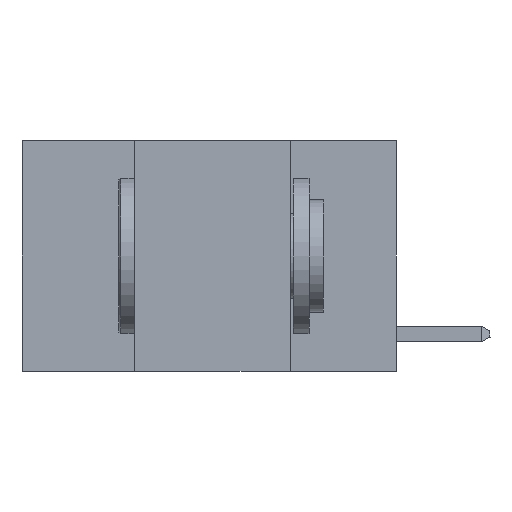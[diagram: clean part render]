
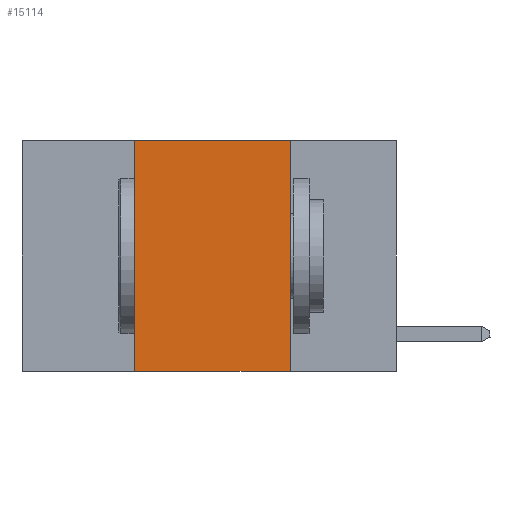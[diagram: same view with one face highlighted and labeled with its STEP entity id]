
A CAD part, left-side view. The second image highlights one B-rep face of the part: STEP entity #15114.
In plain terms, the highlighted planar face has unit normal (-1, 0, 0).
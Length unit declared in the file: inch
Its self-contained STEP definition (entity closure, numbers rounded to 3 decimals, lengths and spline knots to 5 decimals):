
#114 = CARTESIAN_POINT ( 'NONE',  ( 0., 0.6, 0. ) ) ;
#637 = AXIS2_PLACEMENT_3D ( 'NONE', #8810, #13200, #4374 ) ;
#962 = VECTOR ( 'NONE', #7090, 39.37008 ) ;
#1619 = LINE ( 'NONE', #114, #12970 ) ;
#2044 = ORIENTED_EDGE ( 'NONE', *, *, #5881, .F. ) ;
#2088 = ORIENTED_EDGE ( 'NONE', *, *, #13808, .F. ) ;
#2373 = CARTESIAN_POINT ( 'NONE',  ( 0., 0.42, 0. ) ) ;
#2862 = PLANE ( 'NONE',  #637 ) ;
#3493 = LINE ( 'NONE', #15088, #14798 ) ;
#4015 = CARTESIAN_POINT ( 'NONE',  ( 0., 0.17, -0.37 ) ) ;
#4357 = DIRECTION ( 'NONE',  ( 0., 0., -1. ) ) ;
#4374 = DIRECTION ( 'NONE',  ( 0., 0., -1. ) ) ;
#5881 = EDGE_CURVE ( 'NONE', #11765, #14217, #1619, .T. ) ;
#6009 = ORIENTED_EDGE ( 'NONE', *, *, #18899, .T. ) ;
#6260 = FACE_OUTER_BOUND ( 'NONE', #18002, .T. ) ;
#7090 = DIRECTION ( 'NONE',  ( 0., -1., 0. ) ) ;
#7382 = ORIENTED_EDGE ( 'NONE', *, *, #10337, .F. ) ;
#8810 = CARTESIAN_POINT ( 'NONE',  ( 0., 0.6, 0. ) ) ;
#9285 = VERTEX_POINT ( 'NONE', #10304 ) ;
#10304 = CARTESIAN_POINT ( 'NONE',  ( 0., 0.42, -0.37 ) ) ;
#10337 = EDGE_CURVE ( 'NONE', #9285, #11765, #3493, .T. ) ;
#10565 = DIRECTION ( 'NONE',  ( 0., -1., 0. ) ) ;
#11030 = LINE ( 'NONE', #11717, #18328 ) ;
#11717 = CARTESIAN_POINT ( 'NONE',  ( 0., 0.17, 0. ) ) ;
#11765 = VERTEX_POINT ( 'NONE', #2373 ) ;
#12212 = DIRECTION ( 'NONE',  ( 0., 0., 1. ) ) ;
#12437 = VERTEX_POINT ( 'NONE', #4015 ) ;
#12662 = CARTESIAN_POINT ( 'NONE',  ( 0., 0.17, 0. ) ) ;
#12970 = VECTOR ( 'NONE', #10565, 39.37008 ) ;
#13200 = DIRECTION ( 'NONE',  ( 1., 0., 0. ) ) ;
#13808 = EDGE_CURVE ( 'NONE', #14217, #12437, #11030, .T. ) ;
#14217 = VERTEX_POINT ( 'NONE', #12662 ) ;
#14373 = CARTESIAN_POINT ( 'NONE',  ( 0., 0.6, -0.37 ) ) ;
#14798 = VECTOR ( 'NONE', #12212, 39.37008 ) ;
#15088 = CARTESIAN_POINT ( 'NONE',  ( 0., 0.42, 0. ) ) ;
#15114 = ADVANCED_FACE ( 'NONE', ( #6260 ), #2862, .F. ) ;
#15739 = LINE ( 'NONE', #14373, #962 ) ;
#18002 = EDGE_LOOP ( 'NONE', ( #2088, #2044, #7382, #6009 ) ) ;
#18328 = VECTOR ( 'NONE', #4357, 39.37008 ) ;
#18899 = EDGE_CURVE ( 'NONE', #9285, #12437, #15739, .T. ) ;
